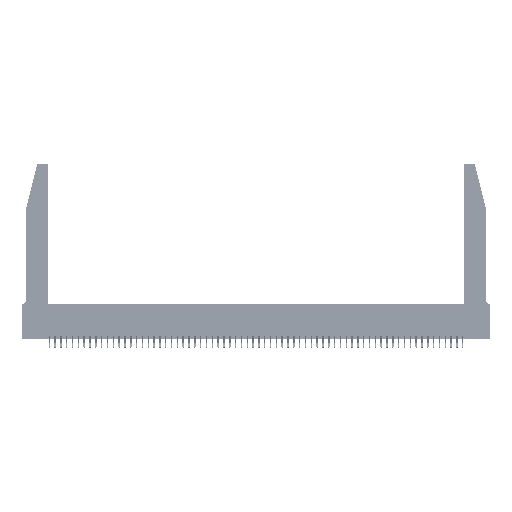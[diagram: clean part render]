
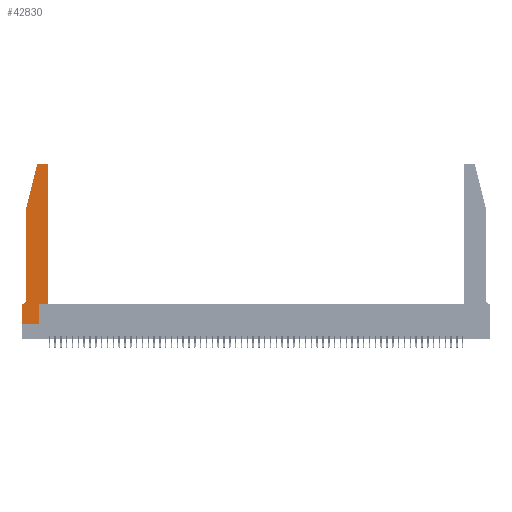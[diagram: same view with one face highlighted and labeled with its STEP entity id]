
A CAD part, top view. The second image highlights one B-rep face of the part: STEP entity #42830.
In plain terms, the highlighted planar face has unit normal (0, 0, 1).
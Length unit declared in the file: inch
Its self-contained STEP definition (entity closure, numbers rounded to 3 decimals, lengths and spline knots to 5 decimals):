
#906 = DIRECTION ( 'NONE',  ( 1., 0., 0. ) ) ;
#2788 = CARTESIAN_POINT ( 'NONE',  ( 0.2865, 0.35, 0.37 ) ) ;
#3142 = EDGE_CURVE ( 'NONE', #48563, #17521, #37404, .T. ) ;
#4143 = LINE ( 'NONE', #44071, #26490 ) ;
#4470 = DIRECTION ( 'NONE',  ( -1., 0., 0. ) ) ;
#4980 = CARTESIAN_POINT ( 'NONE',  ( 0.4505, 0.35, 0.37 ) ) ;
#5774 = LINE ( 'NONE', #2788, #39764 ) ;
#6403 = VECTOR ( 'NONE', #55547, 39.37008 ) ;
#7367 = VERTEX_POINT ( 'NONE', #47590 ) ;
#7493 = VECTOR ( 'NONE', #15700, 39.37008 ) ;
#8156 = ORIENTED_EDGE ( 'NONE', *, *, #17921, .T. ) ;
#8779 = PLANE ( 'NONE',  #40170 ) ;
#8976 = DIRECTION ( 'NONE',  ( 0., 0., 1. ) ) ;
#9360 = ORIENTED_EDGE ( 'NONE', *, *, #3142, .T. ) ;
#10726 = CARTESIAN_POINT ( 'NONE',  ( 0.0755, 2., 0.37 ) ) ;
#12218 = ORIENTED_EDGE ( 'NONE', *, *, #46534, .T. ) ;
#14180 = AXIS2_PLACEMENT_3D ( 'NONE', #18205, #49009, #22653 ) ;
#14818 = CARTESIAN_POINT ( 'NONE',  ( 0.4205, 2.72, 0.37 ) ) ;
#15700 = DIRECTION ( 'NONE',  ( 0., 1., 0. ) ) ;
#16973 = VERTEX_POINT ( 'NONE', #46047 ) ;
#17459 = EDGE_LOOP ( 'NONE', ( #45908, #35049, #50844, #18300, #27226, #28756, #48033, #9360, #12218, #28184, #33840, #8156 ) ) ;
#17521 = VERTEX_POINT ( 'NONE', #38666 ) ;
#17816 = EDGE_CURVE ( 'NONE', #56040, #25885, #28286, .T. ) ;
#17921 = EDGE_CURVE ( 'NONE', #7367, #18084, #34463, .T. ) ;
#18084 = VERTEX_POINT ( 'NONE', #46668 ) ;
#18205 = CARTESIAN_POINT ( 'NONE',  ( 0.0055, 0.42, 0.37 ) ) ;
#18287 = LINE ( 'NONE', #20331, #6403 ) ;
#18300 = ORIENTED_EDGE ( 'NONE', *, *, #18905, .T. ) ;
#18477 = CIRCLE ( 'NONE', #14180, 0.07 ) ;
#18598 = VECTOR ( 'NONE', #18654, 39.37008 ) ;
#18654 = DIRECTION ( 'NONE',  ( 1., 0., 0. ) ) ;
#18905 = EDGE_CURVE ( 'NONE', #25885, #16973, #53562, .T. ) ;
#19113 = CIRCLE ( 'NONE', #29801, 0.03 ) ;
#19293 = DIRECTION ( 'NONE',  ( 1., 0., 0. ) ) ;
#20331 = CARTESIAN_POINT ( 'NONE',  ( 0.2605, 2.75, 0.37 ) ) ;
#20698 = LINE ( 'NONE', #48595, #54430 ) ;
#20774 = DIRECTION ( 'NONE',  ( 0., 1., 0. ) ) ;
#21343 = CARTESIAN_POINT ( 'NONE',  ( 0., 0., 0.37 ) ) ;
#22222 = EDGE_CURVE ( 'NONE', #23728, #48563, #4143, .T. ) ;
#22653 = DIRECTION ( 'NONE',  ( -1., 0., 0. ) ) ;
#22772 = CARTESIAN_POINT ( 'NONE',  ( 0.284, 2.75, 0.37 ) ) ;
#23373 = CARTESIAN_POINT ( 'NONE',  ( 0., 0.35, 0.37 ) ) ;
#23728 = VERTEX_POINT ( 'NONE', #23373 ) ;
#24988 = EDGE_CURVE ( 'NONE', #16973, #35863, #18477, .T. ) ;
#25678 = VECTOR ( 'NONE', #43528, 39.37008 ) ;
#25885 = VERTEX_POINT ( 'NONE', #10726 ) ;
#26490 = VECTOR ( 'NONE', #48475, 39.37008 ) ;
#27226 = ORIENTED_EDGE ( 'NONE', *, *, #24988, .T. ) ;
#27707 = DIRECTION ( 'NONE',  ( 0., 0., 1. ) ) ;
#28184 = ORIENTED_EDGE ( 'NONE', *, *, #34342, .T. ) ;
#28286 = LINE ( 'NONE', #36128, #50270 ) ;
#28756 = ORIENTED_EDGE ( 'NONE', *, *, #36525, .T. ) ;
#29801 = AXIS2_PLACEMENT_3D ( 'NONE', #54018, #27707, #906 ) ;
#30230 = DIRECTION ( 'NONE',  ( 0., -1., 0. ) ) ;
#30369 = LINE ( 'NONE', #4980, #18598 ) ;
#31975 = CARTESIAN_POINT ( 'NONE',  ( 0.25487, 2.72718, 0.37 ) ) ;
#33840 = ORIENTED_EDGE ( 'NONE', *, *, #56258, .T. ) ;
#34342 = EDGE_CURVE ( 'NONE', #42453, #55872, #30369, .T. ) ;
#34463 = CIRCLE ( 'NONE', #43353, 0.03 ) ;
#35049 = ORIENTED_EDGE ( 'NONE', *, *, #54082, .T. ) ;
#35462 = CARTESIAN_POINT ( 'NONE',  ( 0.4505, 0.35, 0.37 ) ) ;
#35532 = CARTESIAN_POINT ( 'NONE',  ( 0., 0.35, 0.37 ) ) ;
#35863 = VERTEX_POINT ( 'NONE', #47330 ) ;
#36128 = CARTESIAN_POINT ( 'NONE',  ( 0.0755, 2., 0.37 ) ) ;
#36525 = EDGE_CURVE ( 'NONE', #35863, #23728, #20698, .T. ) ;
#37404 = LINE ( 'NONE', #21343, #25678 ) ;
#37553 = CARTESIAN_POINT ( 'NONE',  ( 0.4505, 0.35, 0.37 ) ) ;
#38528 = VERTEX_POINT ( 'NONE', #22772 ) ;
#38666 = CARTESIAN_POINT ( 'NONE',  ( 0.2865, 0., 0.37 ) ) ;
#39764 = VECTOR ( 'NONE', #20774, 39.37008 ) ;
#39933 = DIRECTION ( 'NONE',  ( 1., 0., 0. ) ) ;
#40170 = AXIS2_PLACEMENT_3D ( 'NONE', #35532, #8976, #39933 ) ;
#40527 = DIRECTION ( 'NONE',  ( -0.239, -0.971, 0. ) ) ;
#40861 = FACE_OUTER_BOUND ( 'NONE', #17459, .T. ) ;
#41927 = VECTOR ( 'NONE', #30230, 39.37008 ) ;
#42453 = VERTEX_POINT ( 'NONE', #45549 ) ;
#42830 = ADVANCED_FACE ( 'NONE', ( #40861 ), #8779, .T. ) ;
#43353 = AXIS2_PLACEMENT_3D ( 'NONE', #14818, #45701, #19293 ) ;
#43528 = DIRECTION ( 'NONE',  ( 1., 0., 0. ) ) ;
#43589 = CARTESIAN_POINT ( 'NONE',  ( 0., 0., 0.37 ) ) ;
#44071 = CARTESIAN_POINT ( 'NONE',  ( 0., 0., 0.37 ) ) ;
#45549 = CARTESIAN_POINT ( 'NONE',  ( 0.2865, 0.35, 0.37 ) ) ;
#45701 = DIRECTION ( 'NONE',  ( 0., 0., 1. ) ) ;
#45908 = ORIENTED_EDGE ( 'NONE', *, *, #47177, .T. ) ;
#46047 = CARTESIAN_POINT ( 'NONE',  ( 0.0755, 0.42, 0.37 ) ) ;
#46534 = EDGE_CURVE ( 'NONE', #17521, #42453, #5774, .T. ) ;
#46668 = CARTESIAN_POINT ( 'NONE',  ( 0.4205, 2.75, 0.37 ) ) ;
#47177 = EDGE_CURVE ( 'NONE', #18084, #38528, #18287, .T. ) ;
#47330 = CARTESIAN_POINT ( 'NONE',  ( 0.0055, 0.35, 0.37 ) ) ;
#47590 = CARTESIAN_POINT ( 'NONE',  ( 0.4505, 2.72, 0.37 ) ) ;
#47721 = CARTESIAN_POINT ( 'NONE',  ( 0.0755, 2., 0.37 ) ) ;
#48033 = ORIENTED_EDGE ( 'NONE', *, *, #22222, .T. ) ;
#48475 = DIRECTION ( 'NONE',  ( 0., -1., 0. ) ) ;
#48563 = VERTEX_POINT ( 'NONE', #43589 ) ;
#48595 = CARTESIAN_POINT ( 'NONE',  ( 0.0755, 0.35, 0.37 ) ) ;
#49009 = DIRECTION ( 'NONE',  ( 0., 0., -1. ) ) ;
#50270 = VECTOR ( 'NONE', #40527, 39.37008 ) ;
#50844 = ORIENTED_EDGE ( 'NONE', *, *, #17816, .T. ) ;
#53562 = LINE ( 'NONE', #47721, #41927 ) ;
#54018 = CARTESIAN_POINT ( 'NONE',  ( 0.284, 2.72, 0.37 ) ) ;
#54082 = EDGE_CURVE ( 'NONE', #38528, #56040, #19113, .T. ) ;
#54430 = VECTOR ( 'NONE', #4470, 39.37008 ) ;
#54484 = LINE ( 'NONE', #37553, #7493 ) ;
#55547 = DIRECTION ( 'NONE',  ( -1., 0., 0. ) ) ;
#55872 = VERTEX_POINT ( 'NONE', #35462 ) ;
#56040 = VERTEX_POINT ( 'NONE', #31975 ) ;
#56258 = EDGE_CURVE ( 'NONE', #55872, #7367, #54484, .T. ) ;
